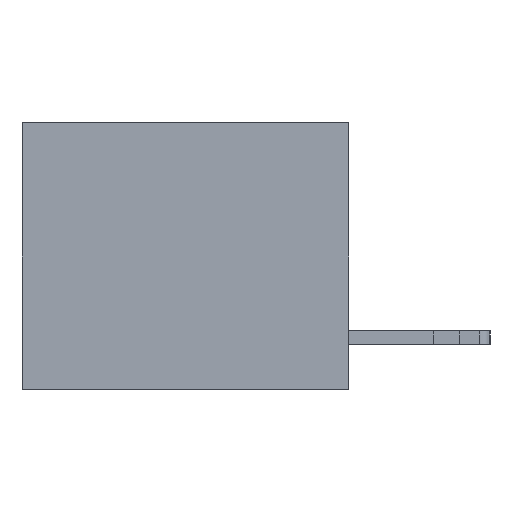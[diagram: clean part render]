
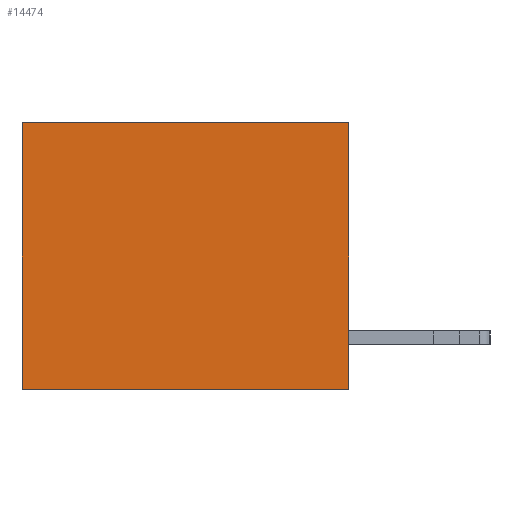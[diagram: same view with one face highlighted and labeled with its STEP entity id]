
A CAD part, left-side view. The second image highlights one B-rep face of the part: STEP entity #14474.
In plain terms, the highlighted planar face has unit normal (-1, 0, 0).
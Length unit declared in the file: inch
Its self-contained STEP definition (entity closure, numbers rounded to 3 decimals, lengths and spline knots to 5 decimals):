
#399 = EDGE_CURVE ( 'NONE', #5093, #20542, #12755, .T. ) ;
#2224 = DIRECTION ( 'NONE',  ( 1., 0., 0. ) ) ;
#2437 = ORIENTED_EDGE ( 'NONE', *, *, #9374, .T. ) ;
#2712 = CARTESIAN_POINT ( 'NONE',  ( 0.3165, 0.6, -0.49 ) ) ;
#2851 = VECTOR ( 'NONE', #4418, 39.37008 ) ;
#3931 = EDGE_LOOP ( 'NONE', ( #2437, #10250, #22178, #10981 ) ) ;
#4418 = DIRECTION ( 'NONE',  ( 0., 0., -1. ) ) ;
#5093 = VERTEX_POINT ( 'NONE', #23431 ) ;
#5551 = DIRECTION ( 'NONE',  ( 0., 1., 0. ) ) ;
#6304 = VECTOR ( 'NONE', #12116, 39.37008 ) ;
#7121 = FACE_OUTER_BOUND ( 'NONE', #3931, .T. ) ;
#7397 = LINE ( 'NONE', #12191, #2851 ) ;
#7519 = EDGE_CURVE ( 'NONE', #13200, #15488, #9461, .T. ) ;
#8659 = AXIS2_PLACEMENT_3D ( 'NONE', #9987, #2224, #15900 ) ;
#8743 = CARTESIAN_POINT ( 'NONE',  ( 0.3165, 0., -0.49 ) ) ;
#9374 = EDGE_CURVE ( 'NONE', #20542, #15488, #13230, .T. ) ;
#9461 = LINE ( 'NONE', #8743, #21393 ) ;
#9987 = CARTESIAN_POINT ( 'NONE',  ( 0.3165, 0., -0.49 ) ) ;
#10250 = ORIENTED_EDGE ( 'NONE', *, *, #7519, .F. ) ;
#10981 = ORIENTED_EDGE ( 'NONE', *, *, #399, .T. ) ;
#11949 = CARTESIAN_POINT ( 'NONE',  ( 0.3165, 0.6, -0.49 ) ) ;
#12116 = DIRECTION ( 'NONE',  ( 0., 1., 0. ) ) ;
#12191 = CARTESIAN_POINT ( 'NONE',  ( 0.3165, 0., -0.49 ) ) ;
#12755 = LINE ( 'NONE', #21736, #6304 ) ;
#12787 = DIRECTION ( 'NONE',  ( 0., 0., -1. ) ) ;
#13200 = VERTEX_POINT ( 'NONE', #14667 ) ;
#13230 = LINE ( 'NONE', #2712, #23009 ) ;
#14474 = ADVANCED_FACE ( 'NONE', ( #7121 ), #21666, .F. ) ;
#14667 = CARTESIAN_POINT ( 'NONE',  ( 0.3165, 0., -0.49 ) ) ;
#15488 = VERTEX_POINT ( 'NONE', #11949 ) ;
#15900 = DIRECTION ( 'NONE',  ( 0., 0., -1. ) ) ;
#20542 = VERTEX_POINT ( 'NONE', #24552 ) ;
#21393 = VECTOR ( 'NONE', #5551, 39.37008 ) ;
#21666 = PLANE ( 'NONE',  #8659 ) ;
#21736 = CARTESIAN_POINT ( 'NONE',  ( 0.3165, 0., 0. ) ) ;
#22178 = ORIENTED_EDGE ( 'NONE', *, *, #22754, .F. ) ;
#22754 = EDGE_CURVE ( 'NONE', #5093, #13200, #7397, .T. ) ;
#23009 = VECTOR ( 'NONE', #12787, 39.37008 ) ;
#23431 = CARTESIAN_POINT ( 'NONE',  ( 0.3165, 0., 0. ) ) ;
#24552 = CARTESIAN_POINT ( 'NONE',  ( 0.3165, 0.6, 0. ) ) ;
